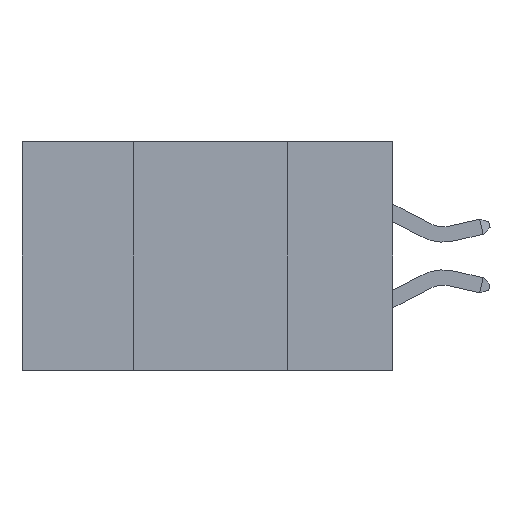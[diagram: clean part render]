
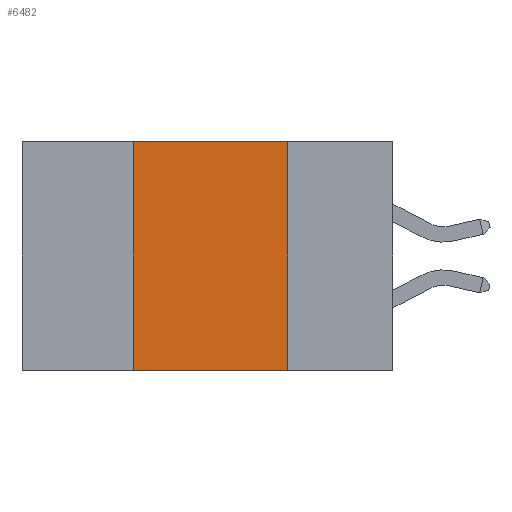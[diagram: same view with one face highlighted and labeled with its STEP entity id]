
A CAD part, left-side view. The second image highlights one B-rep face of the part: STEP entity #6482.
In plain terms, the highlighted planar face has unit normal (-1, 0, 0).
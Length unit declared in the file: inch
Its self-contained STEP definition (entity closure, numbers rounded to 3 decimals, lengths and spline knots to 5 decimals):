
#136 = VERTEX_POINT ( 'NONE', #14900 ) ;
#2186 = LINE ( 'NONE', #5158, #20472 ) ;
#2929 = FACE_OUTER_BOUND ( 'NONE', #8374, .T. ) ;
#3393 = EDGE_CURVE ( 'NONE', #21091, #4711, #10079, .T. ) ;
#3988 = ORIENTED_EDGE ( 'NONE', *, *, #14362, .F. ) ;
#4711 = VERTEX_POINT ( 'NONE', #19630 ) ;
#4957 = EDGE_CURVE ( 'NONE', #10094, #136, #2186, .T. ) ;
#5158 = CARTESIAN_POINT ( 'NONE',  ( 0., 0.6, -0.37 ) ) ;
#6451 = CARTESIAN_POINT ( 'NONE',  ( 0., 0.6, 0. ) ) ;
#6482 = ADVANCED_FACE ( 'NONE', ( #2929 ), #17088, .F. ) ;
#7184 = DIRECTION ( 'NONE',  ( 1., 0., 0. ) ) ;
#8374 = EDGE_LOOP ( 'NONE', ( #3988, #11448, #21353, #12204 ) ) ;
#8869 = LINE ( 'NONE', #19621, #9400 ) ;
#9267 = LINE ( 'NONE', #9339, #17994 ) ;
#9339 = CARTESIAN_POINT ( 'NONE',  ( 0., 0.42, 0. ) ) ;
#9400 = VECTOR ( 'NONE', #21141, 39.37008 ) ;
#10079 = LINE ( 'NONE', #6451, #11102 ) ;
#10094 = VERTEX_POINT ( 'NONE', #10625 ) ;
#10625 = CARTESIAN_POINT ( 'NONE',  ( 0., 0.42, -0.37 ) ) ;
#10828 = EDGE_CURVE ( 'NONE', #10094, #21091, #9267, .T. ) ;
#11102 = VECTOR ( 'NONE', #14777, 39.37008 ) ;
#11448 = ORIENTED_EDGE ( 'NONE', *, *, #3393, .F. ) ;
#11690 = CARTESIAN_POINT ( 'NONE',  ( 0., 0.42, 0. ) ) ;
#12204 = ORIENTED_EDGE ( 'NONE', *, *, #4957, .T. ) ;
#12604 = DIRECTION ( 'NONE',  ( 0., 0., 1. ) ) ;
#13307 = AXIS2_PLACEMENT_3D ( 'NONE', #13838, #7184, #18725 ) ;
#13838 = CARTESIAN_POINT ( 'NONE',  ( 0., 0.6, 0. ) ) ;
#14362 = EDGE_CURVE ( 'NONE', #4711, #136, #8869, .T. ) ;
#14777 = DIRECTION ( 'NONE',  ( 0., -1., 0. ) ) ;
#14900 = CARTESIAN_POINT ( 'NONE',  ( 0., 0.17, -0.37 ) ) ;
#17088 = PLANE ( 'NONE',  #13307 ) ;
#17994 = VECTOR ( 'NONE', #12604, 39.37008 ) ;
#18470 = DIRECTION ( 'NONE',  ( 0., -1., 0. ) ) ;
#18725 = DIRECTION ( 'NONE',  ( 0., 0., -1. ) ) ;
#19621 = CARTESIAN_POINT ( 'NONE',  ( 0., 0.17, 0. ) ) ;
#19630 = CARTESIAN_POINT ( 'NONE',  ( 0., 0.17, 0. ) ) ;
#20472 = VECTOR ( 'NONE', #18470, 39.37008 ) ;
#21091 = VERTEX_POINT ( 'NONE', #11690 ) ;
#21141 = DIRECTION ( 'NONE',  ( 0., 0., -1. ) ) ;
#21353 = ORIENTED_EDGE ( 'NONE', *, *, #10828, .F. ) ;
